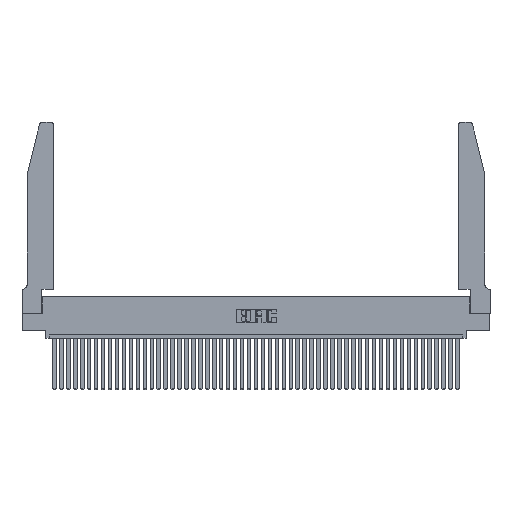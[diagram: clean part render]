
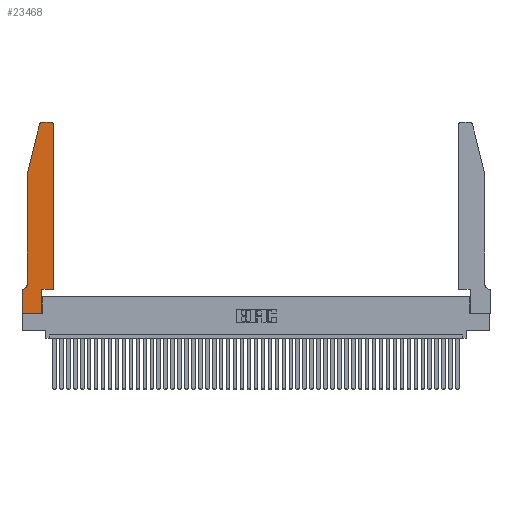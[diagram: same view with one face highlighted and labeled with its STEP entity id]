
A CAD part, top view. The second image highlights one B-rep face of the part: STEP entity #23468.
In plain terms, the highlighted planar face has unit normal (0, 0, 1).
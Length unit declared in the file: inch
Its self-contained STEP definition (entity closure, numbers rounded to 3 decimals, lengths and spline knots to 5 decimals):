
#60 = DIRECTION ( 'NONE',  ( 1., 0., 0. ) ) ;
#1381 = VECTOR ( 'NONE', #15434, 39.37008 ) ;
#1488 = CARTESIAN_POINT ( 'NONE',  ( 0.2605, 2.75, 0.37 ) ) ;
#1674 = EDGE_CURVE ( 'NONE', #19978, #35264, #20599, .T. ) ;
#1811 = ORIENTED_EDGE ( 'NONE', *, *, #18096, .T. ) ;
#2154 = CARTESIAN_POINT ( 'NONE',  ( 0., 0., 0.37 ) ) ;
#3872 = DIRECTION ( 'NONE',  ( 0., 0., 1. ) ) ;
#4066 = LINE ( 'NONE', #41586, #17009 ) ;
#4134 = PLANE ( 'NONE',  #28964 ) ;
#4936 = CARTESIAN_POINT ( 'NONE',  ( 0.0055, 0.35, 0.37 ) ) ;
#4942 = VECTOR ( 'NONE', #44385, 39.37008 ) ;
#5233 = CARTESIAN_POINT ( 'NONE',  ( 0.2865, 0.35, 0.37 ) ) ;
#5786 = CIRCLE ( 'NONE', #18068, 0.03 ) ;
#6091 = VECTOR ( 'NONE', #17444, 39.37008 ) ;
#6250 = VERTEX_POINT ( 'NONE', #7706 ) ;
#6846 = EDGE_CURVE ( 'NONE', #12327, #19978, #7412, .T. ) ;
#7082 = VECTOR ( 'NONE', #20068, 39.37008 ) ;
#7412 = CIRCLE ( 'NONE', #40123, 0.03 ) ;
#7706 = CARTESIAN_POINT ( 'NONE',  ( 0.2865, 0.35, 0.37 ) ) ;
#8176 = VERTEX_POINT ( 'NONE', #2154 ) ;
#8370 = ORIENTED_EDGE ( 'NONE', *, *, #25182, .T. ) ;
#8442 = VECTOR ( 'NONE', #22713, 39.37008 ) ;
#8495 = CARTESIAN_POINT ( 'NONE',  ( 0.4205, 2.75, 0.37 ) ) ;
#8630 = EDGE_LOOP ( 'NONE', ( #45591, #26896, #1811, #33789, #19508, #15568, #8370, #40702, #36438, #23959, #21168, #28846 ) ) ;
#8696 = DIRECTION ( 'NONE',  ( 1., 0., 0. ) ) ;
#11445 = LINE ( 'NONE', #28930, #12580 ) ;
#12327 = VERTEX_POINT ( 'NONE', #20039 ) ;
#12580 = VECTOR ( 'NONE', #60, 39.37008 ) ;
#13199 = CARTESIAN_POINT ( 'NONE',  ( 0.0755, 2., 0.37 ) ) ;
#13526 = CARTESIAN_POINT ( 'NONE',  ( 0.4205, 2.72, 0.37 ) ) ;
#13730 = LINE ( 'NONE', #13199, #46029 ) ;
#14441 = CARTESIAN_POINT ( 'NONE',  ( 0.2865, 0., 0.37 ) ) ;
#14745 = CARTESIAN_POINT ( 'NONE',  ( 0.25487, 2.72718, 0.37 ) ) ;
#15219 = LINE ( 'NONE', #5233, #8442 ) ;
#15434 = DIRECTION ( 'NONE',  ( 0., -1., 0. ) ) ;
#15568 = ORIENTED_EDGE ( 'NONE', *, *, #45986, .T. ) ;
#16005 = CARTESIAN_POINT ( 'NONE',  ( 0.0055, 0.42, 0.37 ) ) ;
#17009 = VECTOR ( 'NONE', #8696, 39.37008 ) ;
#17167 = DIRECTION ( 'NONE',  ( 1., 0., 0. ) ) ;
#17444 = DIRECTION ( 'NONE',  ( 0., -1., 0. ) ) ;
#18068 = AXIS2_PLACEMENT_3D ( 'NONE', #32556, #3872, #32863 ) ;
#18096 = EDGE_CURVE ( 'NONE', #33213, #19635, #13730, .T. ) ;
#19043 = EDGE_CURVE ( 'NONE', #6250, #43239, #4066, .T. ) ;
#19089 = CARTESIAN_POINT ( 'NONE',  ( 0.0755, 0.35, 0.37 ) ) ;
#19370 = CARTESIAN_POINT ( 'NONE',  ( 0., 0., 0.37 ) ) ;
#19508 = ORIENTED_EDGE ( 'NONE', *, *, #27229, .T. ) ;
#19635 = VERTEX_POINT ( 'NONE', #42370 ) ;
#19652 = DIRECTION ( 'NONE',  ( 0., 0., -1. ) ) ;
#19978 = VERTEX_POINT ( 'NONE', #8495 ) ;
#20039 = CARTESIAN_POINT ( 'NONE',  ( 0.4505, 2.72, 0.37 ) ) ;
#20068 = DIRECTION ( 'NONE',  ( -1., 0., 0. ) ) ;
#20307 = VERTEX_POINT ( 'NONE', #14441 ) ;
#20599 = LINE ( 'NONE', #1488, #7082 ) ;
#20843 = AXIS2_PLACEMENT_3D ( 'NONE', #16005, #19652, #44952 ) ;
#20982 = CARTESIAN_POINT ( 'NONE',  ( 0.4505, 0.35, 0.37 ) ) ;
#21168 = ORIENTED_EDGE ( 'NONE', *, *, #34762, .T. ) ;
#22713 = DIRECTION ( 'NONE',  ( 0., 1., 0. ) ) ;
#23468 = ADVANCED_FACE ( 'NONE', ( #25985 ), #4134, .T. ) ;
#23959 = ORIENTED_EDGE ( 'NONE', *, *, #19043, .T. ) ;
#24542 = CARTESIAN_POINT ( 'NONE',  ( 0.0755, 2., 0.37 ) ) ;
#25182 = EDGE_CURVE ( 'NONE', #30558, #8176, #26204, .T. ) ;
#25985 = FACE_OUTER_BOUND ( 'NONE', #8630, .T. ) ;
#26204 = LINE ( 'NONE', #19370, #1381 ) ;
#26896 = ORIENTED_EDGE ( 'NONE', *, *, #42737, .T. ) ;
#27229 = EDGE_CURVE ( 'NONE', #37982, #28300, #36726, .T. ) ;
#27909 = DIRECTION ( 'NONE',  ( -0.239, -0.971, 0. ) ) ;
#28300 = VERTEX_POINT ( 'NONE', #4936 ) ;
#28417 = CARTESIAN_POINT ( 'NONE',  ( 0., 0.35, 0.37 ) ) ;
#28846 = ORIENTED_EDGE ( 'NONE', *, *, #6846, .T. ) ;
#28930 = CARTESIAN_POINT ( 'NONE',  ( 0., 0., 0.37 ) ) ;
#28964 = AXIS2_PLACEMENT_3D ( 'NONE', #32813, #36762, #29511 ) ;
#29403 = EDGE_CURVE ( 'NONE', #19635, #37982, #38845, .T. ) ;
#29511 = DIRECTION ( 'NONE',  ( 1., 0., 0. ) ) ;
#30003 = EDGE_CURVE ( 'NONE', #8176, #20307, #11445, .T. ) ;
#30558 = VERTEX_POINT ( 'NONE', #28417 ) ;
#32556 = CARTESIAN_POINT ( 'NONE',  ( 0.284, 2.72, 0.37 ) ) ;
#32813 = CARTESIAN_POINT ( 'NONE',  ( 0., 0.35, 0.37 ) ) ;
#32863 = DIRECTION ( 'NONE',  ( 1., 0., 0. ) ) ;
#33213 = VERTEX_POINT ( 'NONE', #14745 ) ;
#33726 = LINE ( 'NONE', #19089, #4942 ) ;
#33789 = ORIENTED_EDGE ( 'NONE', *, *, #29403, .T. ) ;
#34762 = EDGE_CURVE ( 'NONE', #43239, #12327, #38193, .T. ) ;
#35264 = VERTEX_POINT ( 'NONE', #41041 ) ;
#36438 = ORIENTED_EDGE ( 'NONE', *, *, #38221, .T. ) ;
#36458 = VECTOR ( 'NONE', #46308, 39.37008 ) ;
#36726 = CIRCLE ( 'NONE', #20843, 0.07 ) ;
#36762 = DIRECTION ( 'NONE',  ( 0., 0., 1. ) ) ;
#37982 = VERTEX_POINT ( 'NONE', #43475 ) ;
#38193 = LINE ( 'NONE', #20982, #36458 ) ;
#38221 = EDGE_CURVE ( 'NONE', #20307, #6250, #15219, .T. ) ;
#38680 = DIRECTION ( 'NONE',  ( 0., 0., 1. ) ) ;
#38845 = LINE ( 'NONE', #24542, #6091 ) ;
#40123 = AXIS2_PLACEMENT_3D ( 'NONE', #13526, #38680, #17167 ) ;
#40702 = ORIENTED_EDGE ( 'NONE', *, *, #30003, .T. ) ;
#41041 = CARTESIAN_POINT ( 'NONE',  ( 0.284, 2.75, 0.37 ) ) ;
#41586 = CARTESIAN_POINT ( 'NONE',  ( 0.4505, 0.35, 0.37 ) ) ;
#42370 = CARTESIAN_POINT ( 'NONE',  ( 0.0755, 2., 0.37 ) ) ;
#42737 = EDGE_CURVE ( 'NONE', #35264, #33213, #5786, .T. ) ;
#43239 = VERTEX_POINT ( 'NONE', #46621 ) ;
#43475 = CARTESIAN_POINT ( 'NONE',  ( 0.0755, 0.42, 0.37 ) ) ;
#44385 = DIRECTION ( 'NONE',  ( -1., 0., 0. ) ) ;
#44952 = DIRECTION ( 'NONE',  ( -1., 0., 0. ) ) ;
#45591 = ORIENTED_EDGE ( 'NONE', *, *, #1674, .T. ) ;
#45986 = EDGE_CURVE ( 'NONE', #28300, #30558, #33726, .T. ) ;
#46029 = VECTOR ( 'NONE', #27909, 39.37008 ) ;
#46308 = DIRECTION ( 'NONE',  ( 0., 1., 0. ) ) ;
#46621 = CARTESIAN_POINT ( 'NONE',  ( 0.4505, 0.35, 0.37 ) ) ;
